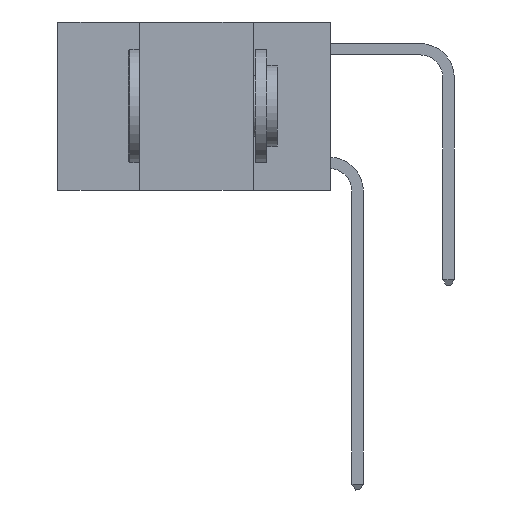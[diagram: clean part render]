
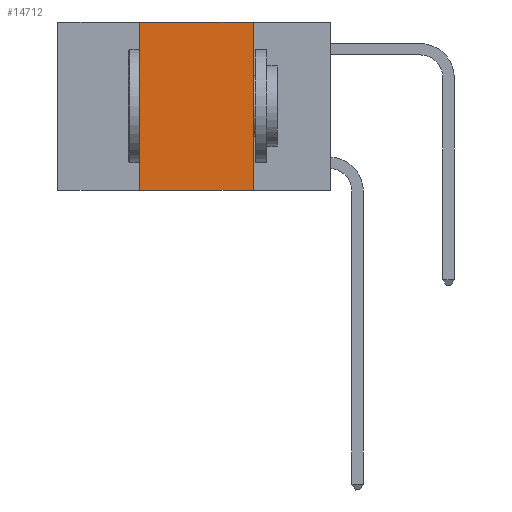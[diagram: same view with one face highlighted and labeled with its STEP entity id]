
A CAD part, left-side view. The second image highlights one B-rep face of the part: STEP entity #14712.
In plain terms, the highlighted planar face has unit normal (-1, 0, 0).
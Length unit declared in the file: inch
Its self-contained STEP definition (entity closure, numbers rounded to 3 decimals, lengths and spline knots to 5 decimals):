
#2629 = PLANE ( 'NONE',  #7365 ) ;
#2652 = LINE ( 'NONE', #9958, #12906 ) ;
#3166 = LINE ( 'NONE', #12517, #16067 ) ;
#3231 = CARTESIAN_POINT ( 'NONE',  ( 0., 0.42, -0.37 ) ) ;
#5183 = CARTESIAN_POINT ( 'NONE',  ( 0., 0.17, 0. ) ) ;
#5352 = VERTEX_POINT ( 'NONE', #3231 ) ;
#6582 = EDGE_CURVE ( 'NONE', #5352, #22204, #14116, .T. ) ;
#6752 = DIRECTION ( 'NONE',  ( 0., -1., 0. ) ) ;
#6869 = DIRECTION ( 'NONE',  ( 0., 0., -1. ) ) ;
#7365 = AXIS2_PLACEMENT_3D ( 'NONE', #16908, #11385, #20828 ) ;
#8982 = CARTESIAN_POINT ( 'NONE',  ( 0., 0.17, 0. ) ) ;
#9376 = ORIENTED_EDGE ( 'NONE', *, *, #11110, .F. ) ;
#9958 = CARTESIAN_POINT ( 'NONE',  ( 0., 0.6, 0. ) ) ;
#10798 = EDGE_LOOP ( 'NONE', ( #9376, #12835, #16234, #17911 ) ) ;
#11110 = EDGE_CURVE ( 'NONE', #18777, #12737, #13961, .T. ) ;
#11112 = EDGE_CURVE ( 'NONE', #5352, #12737, #3166, .T. ) ;
#11385 = DIRECTION ( 'NONE',  ( 1., 0., 0. ) ) ;
#12324 = CARTESIAN_POINT ( 'NONE',  ( 0., 0.42, 0. ) ) ;
#12517 = CARTESIAN_POINT ( 'NONE',  ( 0., 0.6, -0.37 ) ) ;
#12737 = VERTEX_POINT ( 'NONE', #17087 ) ;
#12835 = ORIENTED_EDGE ( 'NONE', *, *, #18543, .F. ) ;
#12906 = VECTOR ( 'NONE', #15471, 39.37008 ) ;
#13389 = VECTOR ( 'NONE', #6869, 39.37008 ) ;
#13961 = LINE ( 'NONE', #5183, #13389 ) ;
#14116 = LINE ( 'NONE', #12324, #18634 ) ;
#14712 = ADVANCED_FACE ( 'NONE', ( #18579 ), #2629, .F. ) ;
#15471 = DIRECTION ( 'NONE',  ( 0., -1., 0. ) ) ;
#16067 = VECTOR ( 'NONE', #6752, 39.37008 ) ;
#16234 = ORIENTED_EDGE ( 'NONE', *, *, #6582, .F. ) ;
#16908 = CARTESIAN_POINT ( 'NONE',  ( 0., 0.6, 0. ) ) ;
#17087 = CARTESIAN_POINT ( 'NONE',  ( 0., 0.17, -0.37 ) ) ;
#17911 = ORIENTED_EDGE ( 'NONE', *, *, #11112, .T. ) ;
#18543 = EDGE_CURVE ( 'NONE', #22204, #18777, #2652, .T. ) ;
#18579 = FACE_OUTER_BOUND ( 'NONE', #10798, .T. ) ;
#18634 = VECTOR ( 'NONE', #19613, 39.37008 ) ;
#18777 = VERTEX_POINT ( 'NONE', #8982 ) ;
#19613 = DIRECTION ( 'NONE',  ( 0., 0., 1. ) ) ;
#20828 = DIRECTION ( 'NONE',  ( 0., 0., -1. ) ) ;
#20891 = CARTESIAN_POINT ( 'NONE',  ( 0., 0.42, 0. ) ) ;
#22204 = VERTEX_POINT ( 'NONE', #20891 ) ;
